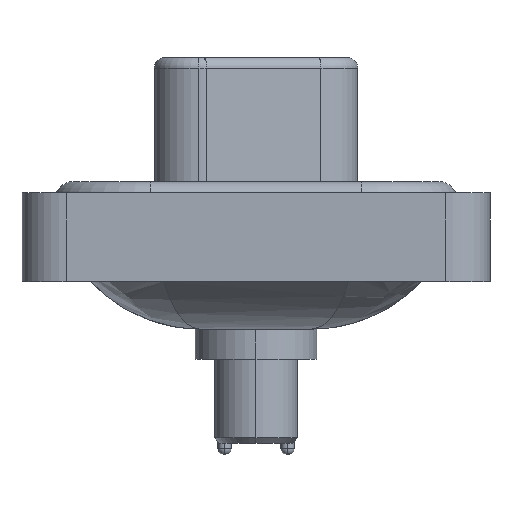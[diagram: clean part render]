
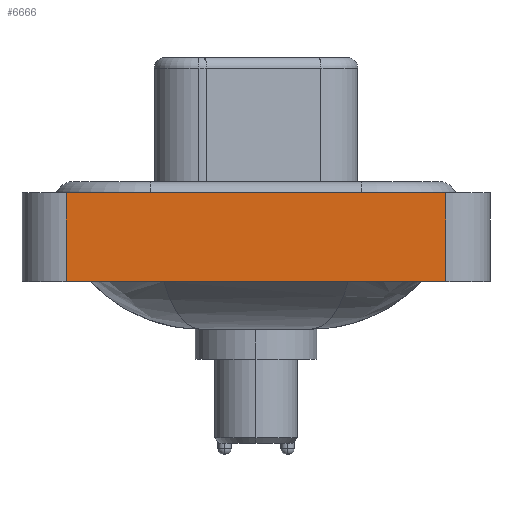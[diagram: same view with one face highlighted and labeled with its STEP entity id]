
A CAD part, left-side view. The second image highlights one B-rep face of the part: STEP entity #6666.
In plain terms, the highlighted planar face has unit normal (-1, 0, 0).
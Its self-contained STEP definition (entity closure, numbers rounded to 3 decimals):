
#1313 = LINE ( 'NONE', #22684, #4060 ) ;
#1381 = CARTESIAN_POINT ( 'NONE',  ( -7.35, -8.55, 0.4 ) ) ;
#1388 = ORIENTED_EDGE ( 'NONE', *, *, #7099, .F. ) ;
#1460 = EDGE_CURVE ( 'NONE', #10844, #3454, #12966, .T. ) ;
#2617 = DIRECTION ( 'NONE',  ( -1., 0., 0. ) ) ;
#3305 = VERTEX_POINT ( 'NONE', #1381 ) ;
#3454 = VERTEX_POINT ( 'NONE', #20518 ) ;
#4048 = AXIS2_PLACEMENT_3D ( 'NONE', #22008, #2617, #18185 ) ;
#4060 = VECTOR ( 'NONE', #6584, 1000. ) ;
#4381 = PLANE ( 'NONE',  #4048 ) ;
#5042 = VERTEX_POINT ( 'NONE', #22712 ) ;
#5437 = EDGE_CURVE ( 'NONE', #5042, #3305, #17012, .T. ) ;
#5778 = FACE_OUTER_BOUND ( 'NONE', #22223, .T. ) ;
#6584 = DIRECTION ( 'NONE',  ( 0., 0., 1. ) ) ;
#6666 = ADVANCED_FACE ( 'NONE', ( #5778 ), #4381, .T. ) ;
#7099 = EDGE_CURVE ( 'NONE', #10844, #5042, #1313, .T. ) ;
#8182 = DIRECTION ( 'NONE',  ( 0., 0., 1. ) ) ;
#8197 = CARTESIAN_POINT ( 'NONE',  ( -7.35, -8.55, 0.4 ) ) ;
#8547 = ORIENTED_EDGE ( 'NONE', *, *, #18147, .T. ) ;
#9354 = DIRECTION ( 'NONE',  ( 0., -1., 0. ) ) ;
#10606 = CARTESIAN_POINT ( 'NONE',  ( -7.35, 8.55, -3.6 ) ) ;
#10844 = VERTEX_POINT ( 'NONE', #10606 ) ;
#11329 = CARTESIAN_POINT ( 'NONE',  ( -7.35, -8.55, -3.6 ) ) ;
#11775 = VECTOR ( 'NONE', #9354, 1000. ) ;
#12966 = LINE ( 'NONE', #11329, #11775 ) ;
#13629 = VECTOR ( 'NONE', #17116, 1000. ) ;
#13632 = CARTESIAN_POINT ( 'NONE',  ( -7.35, -8.55, -3.6 ) ) ;
#13829 = VECTOR ( 'NONE', #8182, 1000. ) ;
#14958 = ORIENTED_EDGE ( 'NONE', *, *, #1460, .T. ) ;
#16872 = LINE ( 'NONE', #13632, #13829 ) ;
#17012 = LINE ( 'NONE', #8197, #13629 ) ;
#17116 = DIRECTION ( 'NONE',  ( 0., -1., 0. ) ) ;
#17744 = ORIENTED_EDGE ( 'NONE', *, *, #5437, .F. ) ;
#18147 = EDGE_CURVE ( 'NONE', #3454, #3305, #16872, .T. ) ;
#18185 = DIRECTION ( 'NONE',  ( 0., 0., 1. ) ) ;
#20518 = CARTESIAN_POINT ( 'NONE',  ( -7.35, -8.55, -3.6 ) ) ;
#22008 = CARTESIAN_POINT ( 'NONE',  ( -7.35, -8.55, -3.6 ) ) ;
#22223 = EDGE_LOOP ( 'NONE', ( #8547, #17744, #1388, #14958 ) ) ;
#22684 = CARTESIAN_POINT ( 'NONE',  ( -7.35, 8.55, -3.6 ) ) ;
#22712 = CARTESIAN_POINT ( 'NONE',  ( -7.35, 8.55, 0.4 ) ) ;
